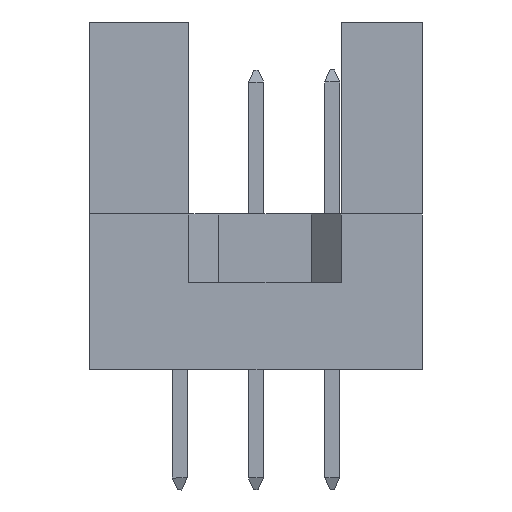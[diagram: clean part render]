
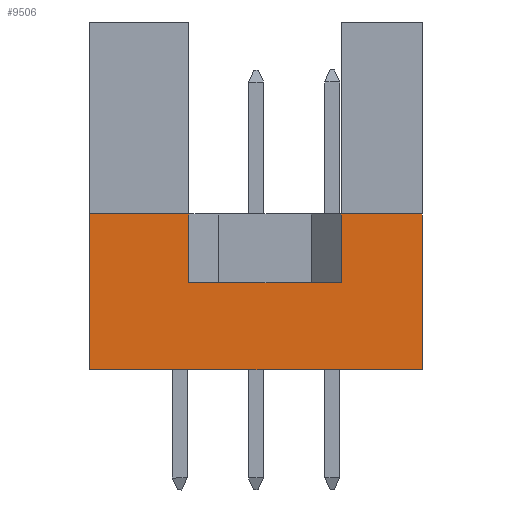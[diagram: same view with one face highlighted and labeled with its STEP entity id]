
A CAD part, left-side view. The second image highlights one B-rep face of the part: STEP entity #9506.
In plain terms, the highlighted planar face has unit normal (-1, 0, 0).
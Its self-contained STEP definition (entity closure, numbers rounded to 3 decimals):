
#187 = CARTESIAN_POINT ( 'NONE',  ( -47.5, 7.79, 5.2 ) ) ;
#391 = LINE ( 'NONE', #9454, #2000 ) ;
#463 = ORIENTED_EDGE ( 'NONE', *, *, #14016, .T. ) ;
#493 = CARTESIAN_POINT ( 'NONE',  ( -47.5, 2.71, 2.9 ) ) ;
#712 = EDGE_CURVE ( 'NONE', #10977, #12698, #4815, .T. ) ;
#1173 = VERTEX_POINT ( 'NONE', #9583 ) ;
#1234 = VERTEX_POINT ( 'NONE', #8640 ) ;
#1767 = DIRECTION ( 'NONE',  ( 0., 0., -1. ) ) ;
#2000 = VECTOR ( 'NONE', #13317, 1000. ) ;
#2046 = DIRECTION ( 'NONE',  ( 0., -1., 0. ) ) ;
#2153 = ORIENTED_EDGE ( 'NONE', *, *, #7619, .T. ) ;
#2155 = CARTESIAN_POINT ( 'NONE',  ( -47.5, 11.1, 5.2 ) ) ;
#2576 = VECTOR ( 'NONE', #15510, 1000. ) ;
#2958 = FACE_OUTER_BOUND ( 'NONE', #11318, .T. ) ;
#3164 = DIRECTION ( 'NONE',  ( 0., -1., 0. ) ) ;
#3319 = LINE ( 'NONE', #11129, #14386 ) ;
#3477 = LINE ( 'NONE', #7475, #7246 ) ;
#4154 = DIRECTION ( 'NONE',  ( 0., 0., 1. ) ) ;
#4522 = VECTOR ( 'NONE', #3164, 1000. ) ;
#4561 = VECTOR ( 'NONE', #10209, 1000. ) ;
#4815 = LINE ( 'NONE', #2155, #4561 ) ;
#5328 = CARTESIAN_POINT ( 'NONE',  ( -47.5, 11.1, 0. ) ) ;
#5434 = LINE ( 'NONE', #10659, #8538 ) ;
#5435 = EDGE_CURVE ( 'NONE', #5743, #13716, #3319, .T. ) ;
#5743 = VERTEX_POINT ( 'NONE', #14851 ) ;
#5880 = ORIENTED_EDGE ( 'NONE', *, *, #10382, .F. ) ;
#6384 = CARTESIAN_POINT ( 'NONE',  ( -47.5, 0., 5.2 ) ) ;
#6605 = LINE ( 'NONE', #5328, #2576 ) ;
#6800 = ORIENTED_EDGE ( 'NONE', *, *, #9876, .T. ) ;
#7003 = CARTESIAN_POINT ( 'NONE',  ( -47.5, 7.79, 2.9 ) ) ;
#7246 = VECTOR ( 'NONE', #15279, 1000. ) ;
#7475 = CARTESIAN_POINT ( 'NONE',  ( -47.5, 0., 0. ) ) ;
#7619 = EDGE_CURVE ( 'NONE', #1173, #12698, #14441, .T. ) ;
#8207 = LINE ( 'NONE', #7003, #4522 ) ;
#8226 = EDGE_CURVE ( 'NONE', #11894, #5743, #5434, .T. ) ;
#8538 = VECTOR ( 'NONE', #4154, 1000. ) ;
#8640 = CARTESIAN_POINT ( 'NONE',  ( -47.5, 0., 0. ) ) ;
#9454 = CARTESIAN_POINT ( 'NONE',  ( -47.5, 11.1, 0. ) ) ;
#9506 = ADVANCED_FACE ( 'NONE', ( #2958 ), #9537, .F. ) ;
#9537 = PLANE ( 'NONE',  #10238 ) ;
#9583 = CARTESIAN_POINT ( 'NONE',  ( -47.5, 7.79, 2.9 ) ) ;
#9876 = EDGE_CURVE ( 'NONE', #12568, #1234, #6605, .T. ) ;
#10209 = DIRECTION ( 'NONE',  ( 0., -1., 0. ) ) ;
#10238 = AXIS2_PLACEMENT_3D ( 'NONE', #12041, #13399, #1767 ) ;
#10382 = EDGE_CURVE ( 'NONE', #12568, #10977, #391, .T. ) ;
#10659 = CARTESIAN_POINT ( 'NONE',  ( -47.5, 2.71, 2.9 ) ) ;
#10977 = VERTEX_POINT ( 'NONE', #12346 ) ;
#11129 = CARTESIAN_POINT ( 'NONE',  ( -47.5, 11.1, 5.2 ) ) ;
#11315 = VECTOR ( 'NONE', #15541, 1000. ) ;
#11318 = EDGE_LOOP ( 'NONE', ( #14246, #2153, #11803, #5880, #6800, #463, #14203, #15370 ) ) ;
#11493 = CARTESIAN_POINT ( 'NONE',  ( -47.5, 11.1, 0. ) ) ;
#11803 = ORIENTED_EDGE ( 'NONE', *, *, #712, .F. ) ;
#11894 = VERTEX_POINT ( 'NONE', #493 ) ;
#12041 = CARTESIAN_POINT ( 'NONE',  ( -47.5, 11.1, 0. ) ) ;
#12346 = CARTESIAN_POINT ( 'NONE',  ( -47.5, 11.1, 5.2 ) ) ;
#12568 = VERTEX_POINT ( 'NONE', #11493 ) ;
#12698 = VERTEX_POINT ( 'NONE', #187 ) ;
#12880 = EDGE_CURVE ( 'NONE', #1173, #11894, #8207, .T. ) ;
#13163 = CARTESIAN_POINT ( 'NONE',  ( -47.5, 7.79, 2.9 ) ) ;
#13317 = DIRECTION ( 'NONE',  ( 0., 0., 1. ) ) ;
#13399 = DIRECTION ( 'NONE',  ( 1., 0., 0. ) ) ;
#13716 = VERTEX_POINT ( 'NONE', #6384 ) ;
#14016 = EDGE_CURVE ( 'NONE', #1234, #13716, #3477, .T. ) ;
#14203 = ORIENTED_EDGE ( 'NONE', *, *, #5435, .F. ) ;
#14246 = ORIENTED_EDGE ( 'NONE', *, *, #12880, .F. ) ;
#14386 = VECTOR ( 'NONE', #2046, 1000. ) ;
#14441 = LINE ( 'NONE', #13163, #11315 ) ;
#14851 = CARTESIAN_POINT ( 'NONE',  ( -47.5, 2.71, 5.2 ) ) ;
#15279 = DIRECTION ( 'NONE',  ( 0., 0., 1. ) ) ;
#15370 = ORIENTED_EDGE ( 'NONE', *, *, #8226, .F. ) ;
#15510 = DIRECTION ( 'NONE',  ( 0., -1., 0. ) ) ;
#15541 = DIRECTION ( 'NONE',  ( 0., 0., 1. ) ) ;
